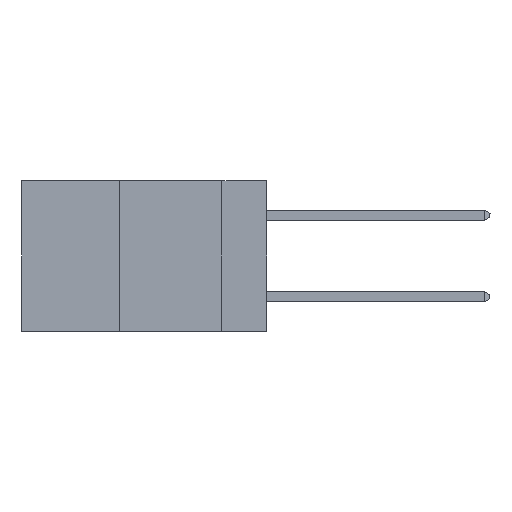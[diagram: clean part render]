
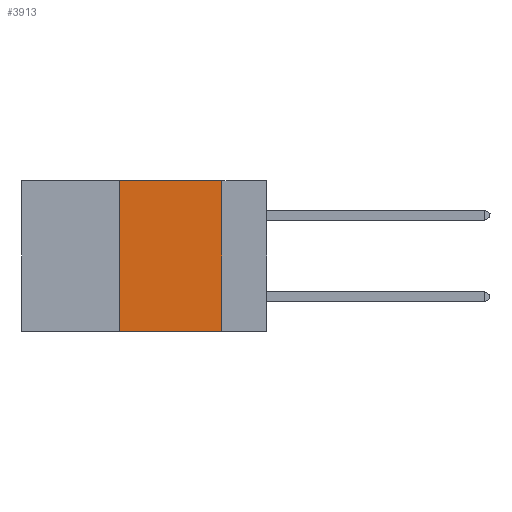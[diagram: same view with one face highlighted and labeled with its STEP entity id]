
A CAD part, left-side view. The second image highlights one B-rep face of the part: STEP entity #3913.
In plain terms, the highlighted planar face has unit normal (-1, 0, 0).
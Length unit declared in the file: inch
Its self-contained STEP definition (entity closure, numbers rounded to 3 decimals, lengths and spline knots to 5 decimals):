
#507 = CARTESIAN_POINT ( 'NONE',  ( 0., 0.36, 0. ) ) ;
#741 = VERTEX_POINT ( 'NONE', #17051 ) ;
#1998 = LINE ( 'NONE', #17635, #5857 ) ;
#2188 = DIRECTION ( 'NONE',  ( 0., 0., 1. ) ) ;
#2606 = VERTEX_POINT ( 'NONE', #7382 ) ;
#3913 = ADVANCED_FACE ( 'NONE', ( #4612 ), #7036, .F. ) ;
#4612 = FACE_OUTER_BOUND ( 'NONE', #9085, .T. ) ;
#4680 = VERTEX_POINT ( 'NONE', #10429 ) ;
#4950 = DIRECTION ( 'NONE',  ( 0., 0., -1. ) ) ;
#5623 = EDGE_CURVE ( 'NONE', #2606, #4680, #1998, .T. ) ;
#5857 = VECTOR ( 'NONE', #4950, 39.37008 ) ;
#7036 = PLANE ( 'NONE',  #13931 ) ;
#7382 = CARTESIAN_POINT ( 'NONE',  ( 0., 0.11, 0. ) ) ;
#7642 = VECTOR ( 'NONE', #2188, 39.37008 ) ;
#7963 = DIRECTION ( 'NONE',  ( 0., -1., 0. ) ) ;
#8406 = CARTESIAN_POINT ( 'NONE',  ( 0., 0.6, 0. ) ) ;
#8744 = VERTEX_POINT ( 'NONE', #12635 ) ;
#9085 = EDGE_LOOP ( 'NONE', ( #15456, #15547, #15730, #16103 ) ) ;
#9789 = LINE ( 'NONE', #8406, #13491 ) ;
#9906 = EDGE_CURVE ( 'NONE', #741, #4680, #19978, .T. ) ;
#10247 = DIRECTION ( 'NONE',  ( 0., 0., -1. ) ) ;
#10429 = CARTESIAN_POINT ( 'NONE',  ( 0., 0.11, -0.37 ) ) ;
#12028 = EDGE_CURVE ( 'NONE', #741, #8744, #16036, .T. ) ;
#12185 = VECTOR ( 'NONE', #7963, 39.37008 ) ;
#12635 = CARTESIAN_POINT ( 'NONE',  ( 0., 0.36, 0. ) ) ;
#13491 = VECTOR ( 'NONE', #14685, 39.37008 ) ;
#13931 = AXIS2_PLACEMENT_3D ( 'NONE', #18095, #19617, #10247 ) ;
#14685 = DIRECTION ( 'NONE',  ( 0., -1., 0. ) ) ;
#15431 = EDGE_CURVE ( 'NONE', #8744, #2606, #9789, .T. ) ;
#15456 = ORIENTED_EDGE ( 'NONE', *, *, #5623, .F. ) ;
#15547 = ORIENTED_EDGE ( 'NONE', *, *, #15431, .F. ) ;
#15730 = ORIENTED_EDGE ( 'NONE', *, *, #12028, .F. ) ;
#16036 = LINE ( 'NONE', #507, #7642 ) ;
#16103 = ORIENTED_EDGE ( 'NONE', *, *, #9906, .T. ) ;
#17051 = CARTESIAN_POINT ( 'NONE',  ( 0., 0.36, -0.37 ) ) ;
#17635 = CARTESIAN_POINT ( 'NONE',  ( 0., 0.11, 0. ) ) ;
#18095 = CARTESIAN_POINT ( 'NONE',  ( 0., 0.6, 0. ) ) ;
#18975 = CARTESIAN_POINT ( 'NONE',  ( 0., 0.6, -0.37 ) ) ;
#19617 = DIRECTION ( 'NONE',  ( 1., 0., 0. ) ) ;
#19978 = LINE ( 'NONE', #18975, #12185 ) ;
